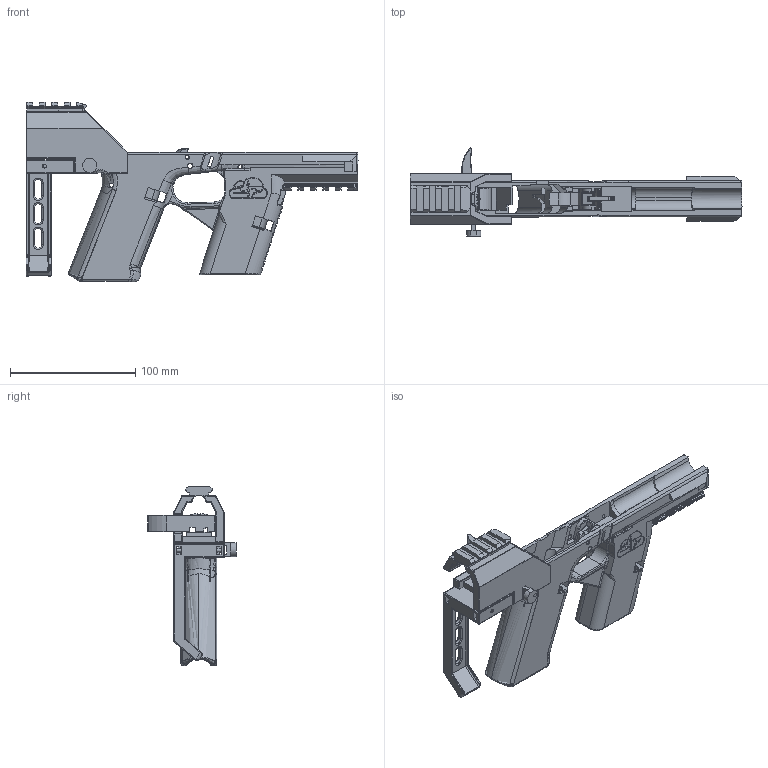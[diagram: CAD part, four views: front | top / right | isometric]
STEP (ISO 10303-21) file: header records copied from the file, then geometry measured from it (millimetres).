
FILE_DESCRIPTION(/* description */ (''),/* implementation_level */ '2;1');
FILE_NAME(/* name */ 'invader_pdw_g17_base.step',/* time_stamp */ '2021-11-17T13:28:59-06:00',/* author */ (''),/* organization */ (''),/* preprocessor_version */ 'ST-DEVELOPER v18.1',/* originating_system */ 'Autodesk Translation Framework v10.10.0.1391',/* authorisation */ '');
FILE_SCHEMA (('AUTOMOTIVE_DESIGN { 1 0 10303 214 3 1 1 }'));
Products named in the file (8): invader_pdw_g17_base; FMDA DD17.2 Assembly.stp; FMDA DD17.2 V1.4 Frame.stp; Brace_Assembly; Brace; Brace_pin; Brace_locking_pin; Charging Handle
Assembly tree (7 placements, depth 3):
  invader_pdw_g17_base
    FMDA DD17.2 Assembly.stp
      FMDA DD17.2 V1.4 Frame.stp
    Brace_Assembly
      Brace
      Brace_pin
    Brace_locking_pin
    Charging Handle
Bounding box: 265.29 x 70.32 x 143.39 mm (x, y, z)
Volume: 232329.4 mm3; surface area: 111841.9 mm2
Topology: 6 solids, 8 shells, 1874 faces, 5240 edges, 3341 vertices
Faces by surface type: plane 835, bspline 476, cylinder 431, torus 69, sphere 54, cone 9
Full cylindrical faces by diameter (mm): 2 x1, 3 x6, 3.1 x4, 3.2 x2, 4 x2, 5 x1, 5.1 x1, 8.4 x1, 10.2 x1, 11 x1
Entity records: 91840 total; most frequent: CARTESIAN_POINT 45739, ORIENTED_EDGE 10436, DIRECTION 8501, EDGE_CURVE 5218, VERTEX_POINT 3342, AXIS2_PLACEMENT_3D 2844, LINE 2813, VECTOR 2813
